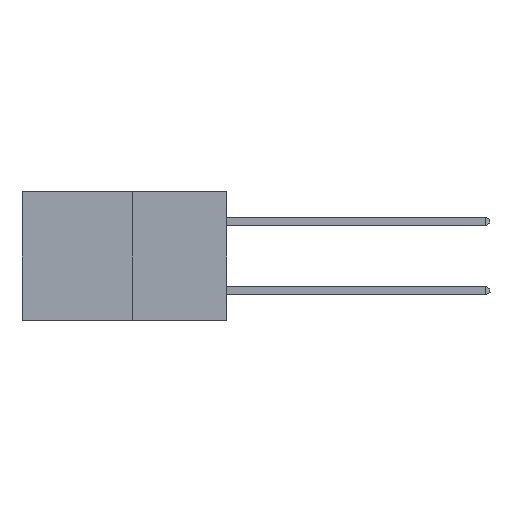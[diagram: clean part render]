
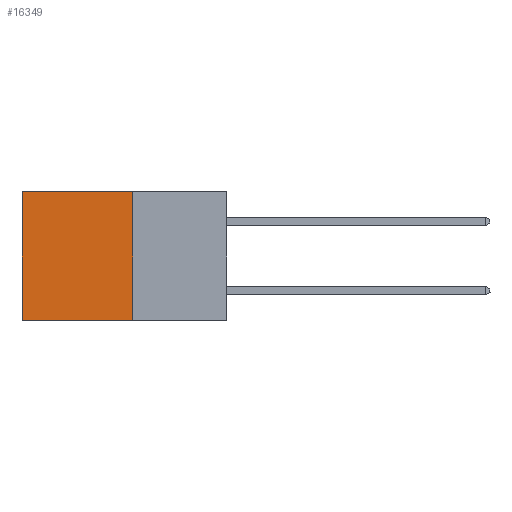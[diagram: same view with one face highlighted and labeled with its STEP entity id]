
A CAD part, left-side view. The second image highlights one B-rep face of the part: STEP entity #16349.
In plain terms, the highlighted planar face has unit normal (-1, 0, 0).
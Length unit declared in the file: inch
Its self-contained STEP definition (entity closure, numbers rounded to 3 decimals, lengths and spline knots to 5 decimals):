
#38 = VERTEX_POINT ( 'NONE', #15567 ) ;
#162 = LINE ( 'NONE', #19453, #19019 ) ;
#851 = PLANE ( 'NONE',  #22200 ) ;
#1107 = VECTOR ( 'NONE', #5115, 39.37008 ) ;
#1391 = EDGE_CURVE ( 'NONE', #8902, #38, #1460, .T. ) ;
#1460 = LINE ( 'NONE', #10670, #15450 ) ;
#1708 = VERTEX_POINT ( 'NONE', #21072 ) ;
#1813 = CARTESIAN_POINT ( 'NONE',  ( 0.277, 0.27, 0. ) ) ;
#2557 = EDGE_CURVE ( 'NONE', #1708, #38, #10292, .T. ) ;
#2724 = DIRECTION ( 'NONE',  ( 0., 0., -1. ) ) ;
#3431 = LINE ( 'NONE', #1813, #11956 ) ;
#3700 = DIRECTION ( 'NONE',  ( 0., 1., 0. ) ) ;
#4760 = ORIENTED_EDGE ( 'NONE', *, *, #2557, .T. ) ;
#5115 = DIRECTION ( 'NONE',  ( 0., 0., -1. ) ) ;
#5193 = CARTESIAN_POINT ( 'NONE',  ( 0.277, 0.59, -0.37 ) ) ;
#8095 = EDGE_CURVE ( 'NONE', #18324, #1708, #3431, .T. ) ;
#8902 = VERTEX_POINT ( 'NONE', #9340 ) ;
#9340 = CARTESIAN_POINT ( 'NONE',  ( 0.277, 0.27, -0.37 ) ) ;
#10090 = CARTESIAN_POINT ( 'NONE',  ( 0.277, 0.27, 0. ) ) ;
#10292 = LINE ( 'NONE', #5193, #1107 ) ;
#10395 = EDGE_LOOP ( 'NONE', ( #4760, #19794, #15003, #17684 ) ) ;
#10446 = DIRECTION ( 'NONE',  ( 0., 1., 0. ) ) ;
#10670 = CARTESIAN_POINT ( 'NONE',  ( 0.277, 0.27, -0.37 ) ) ;
#11956 = VECTOR ( 'NONE', #3700, 39.37008 ) ;
#13652 = DIRECTION ( 'NONE',  ( 1., 0., 0. ) ) ;
#14004 = DIRECTION ( 'NONE',  ( 0., 0., -1. ) ) ;
#15003 = ORIENTED_EDGE ( 'NONE', *, *, #20245, .F. ) ;
#15450 = VECTOR ( 'NONE', #10446, 39.37008 ) ;
#15567 = CARTESIAN_POINT ( 'NONE',  ( 0.277, 0.59, -0.37 ) ) ;
#16349 = ADVANCED_FACE ( 'NONE', ( #16618 ), #851, .F. ) ;
#16618 = FACE_OUTER_BOUND ( 'NONE', #10395, .T. ) ;
#17684 = ORIENTED_EDGE ( 'NONE', *, *, #8095, .T. ) ;
#18324 = VERTEX_POINT ( 'NONE', #10090 ) ;
#19019 = VECTOR ( 'NONE', #14004, 39.37008 ) ;
#19041 = CARTESIAN_POINT ( 'NONE',  ( 0.277, 0.27, -0.37 ) ) ;
#19453 = CARTESIAN_POINT ( 'NONE',  ( 0.277, 0.27, -0.37 ) ) ;
#19794 = ORIENTED_EDGE ( 'NONE', *, *, #1391, .F. ) ;
#20245 = EDGE_CURVE ( 'NONE', #18324, #8902, #162, .T. ) ;
#21072 = CARTESIAN_POINT ( 'NONE',  ( 0.277, 0.59, 0. ) ) ;
#22200 = AXIS2_PLACEMENT_3D ( 'NONE', #19041, #13652, #2724 ) ;
